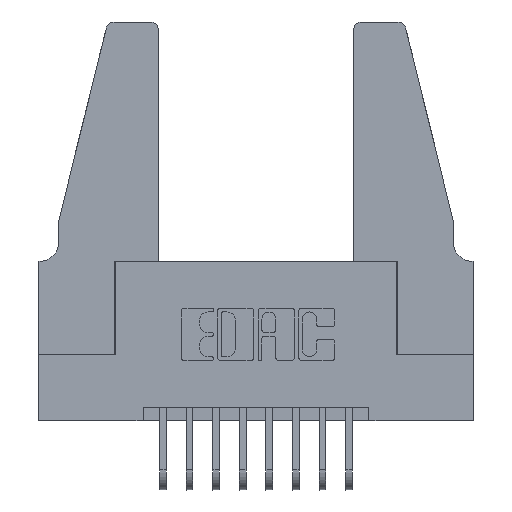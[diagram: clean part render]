
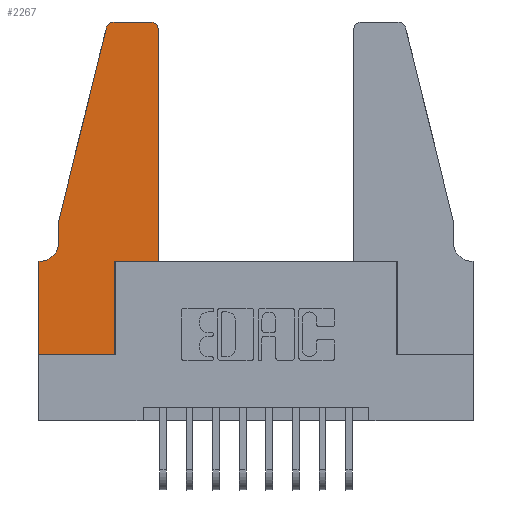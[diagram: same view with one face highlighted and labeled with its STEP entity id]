
A CAD part, top view. The second image highlights one B-rep face of the part: STEP entity #2267.
In plain terms, the highlighted planar face has unit normal (0, 0, 1).
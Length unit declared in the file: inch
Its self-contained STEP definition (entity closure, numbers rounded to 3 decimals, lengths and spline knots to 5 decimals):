
#106 = ORIENTED_EDGE ( 'NONE', *, *, #3151, .T. ) ;
#314 = VECTOR ( 'NONE', #9955, 39.37008 ) ;
#373 = CARTESIAN_POINT ( 'NONE',  ( 0.0755, 0.5, 0.37 ) ) ;
#495 = AXIS2_PLACEMENT_3D ( 'NONE', #718, #8712, #1900 ) ;
#718 = CARTESIAN_POINT ( 'NONE',  ( 0.284, 1.22, 0.37 ) ) ;
#794 = CARTESIAN_POINT ( 'NONE',  ( 0.4205, 1.25, 0.37 ) ) ;
#854 = EDGE_CURVE ( 'NONE', #6997, #4150, #3758, .T. ) ;
#911 = CARTESIAN_POINT ( 'NONE',  ( 0.0755, 0.42, 0.37 ) ) ;
#1144 = EDGE_CURVE ( 'NONE', #11547, #2242, #6611, .T. ) ;
#1324 = ORIENTED_EDGE ( 'NONE', *, *, #3667, .T. ) ;
#1721 = DIRECTION ( 'NONE',  ( 0., -1., 0. ) ) ;
#1776 = EDGE_CURVE ( 'NONE', #3511, #8217, #12428, .T. ) ;
#1794 = EDGE_CURVE ( 'NONE', #9923, #12854, #3394, .T. ) ;
#1900 = DIRECTION ( 'NONE',  ( 1., 0., 0. ) ) ;
#2242 = VERTEX_POINT ( 'NONE', #13448 ) ;
#2267 = ADVANCED_FACE ( 'NONE', ( #3714 ), #11878, .T. ) ;
#2472 = VECTOR ( 'NONE', #1721, 39.37008 ) ;
#3151 = EDGE_CURVE ( 'NONE', #4376, #7071, #13281, .T. ) ;
#3242 = AXIS2_PLACEMENT_3D ( 'NONE', #13270, #6522, #14371 ) ;
#3285 = CARTESIAN_POINT ( 'NONE',  ( 0.2865, 0., 0.37 ) ) ;
#3394 = LINE ( 'NONE', #8948, #9116 ) ;
#3441 = LINE ( 'NONE', #11958, #6100 ) ;
#3511 = VERTEX_POINT ( 'NONE', #8532 ) ;
#3667 = EDGE_CURVE ( 'NONE', #12217, #9923, #12231, .T. ) ;
#3714 = FACE_OUTER_BOUND ( 'NONE', #9520, .T. ) ;
#3758 = LINE ( 'NONE', #11644, #4121 ) ;
#3911 = DIRECTION ( 'NONE',  ( -1., 0., 0. ) ) ;
#3915 = ORIENTED_EDGE ( 'NONE', *, *, #9775, .T. ) ;
#4121 = VECTOR ( 'NONE', #10924, 39.37008 ) ;
#4150 = VERTEX_POINT ( 'NONE', #373 ) ;
#4205 = AXIS2_PLACEMENT_3D ( 'NONE', #7720, #7702, #7655 ) ;
#4224 = EDGE_CURVE ( 'NONE', #4759, #12217, #14110, .T. ) ;
#4376 = VERTEX_POINT ( 'NONE', #794 ) ;
#4382 = CARTESIAN_POINT ( 'NONE',  ( 0.2605, 1.25, 0.37 ) ) ;
#4759 = VERTEX_POINT ( 'NONE', #7159 ) ;
#4923 = ORIENTED_EDGE ( 'NONE', *, *, #854, .T. ) ;
#4986 = CIRCLE ( 'NONE', #3242, 0.03 ) ;
#5549 = ORIENTED_EDGE ( 'NONE', *, *, #1144, .T. ) ;
#5839 = VECTOR ( 'NONE', #13183, 39.37008 ) ;
#5898 = CARTESIAN_POINT ( 'NONE',  ( 0., 0., 0.37 ) ) ;
#5924 = VECTOR ( 'NONE', #11223, 39.37008 ) ;
#5945 = DIRECTION ( 'NONE',  ( 0., -1., 0. ) ) ;
#6098 = LINE ( 'NONE', #13817, #8793 ) ;
#6100 = VECTOR ( 'NONE', #6314, 39.37008 ) ;
#6314 = DIRECTION ( 'NONE',  ( 1., 0., 0. ) ) ;
#6492 = ORIENTED_EDGE ( 'NONE', *, *, #4224, .T. ) ;
#6522 = DIRECTION ( 'NONE',  ( 0., 0., 1. ) ) ;
#6611 = CIRCLE ( 'NONE', #4205, 0.07 ) ;
#6670 = CIRCLE ( 'NONE', #495, 0.03 ) ;
#6826 = EDGE_CURVE ( 'NONE', #12854, #3511, #3441, .T. ) ;
#6924 = VECTOR ( 'NONE', #3911, 39.37008 ) ;
#6997 = VERTEX_POINT ( 'NONE', #12692 ) ;
#7071 = VERTEX_POINT ( 'NONE', #7173 ) ;
#7159 = CARTESIAN_POINT ( 'NONE',  ( 0., 0.35, 0.37 ) ) ;
#7173 = CARTESIAN_POINT ( 'NONE',  ( 0.284, 1.25, 0.37 ) ) ;
#7655 = DIRECTION ( 'NONE',  ( -1., 0., 0. ) ) ;
#7702 = DIRECTION ( 'NONE',  ( 0., 0., -1. ) ) ;
#7720 = CARTESIAN_POINT ( 'NONE',  ( 0.0055, 0.42, 0.37 ) ) ;
#7837 = CARTESIAN_POINT ( 'NONE',  ( 0., 0., 0.37 ) ) ;
#7956 = DIRECTION ( 'NONE',  ( 0., 1., 0. ) ) ;
#8012 = CARTESIAN_POINT ( 'NONE',  ( 0.4505, 1.22, 0.37 ) ) ;
#8217 = VERTEX_POINT ( 'NONE', #8012 ) ;
#8532 = CARTESIAN_POINT ( 'NONE',  ( 0.4505, 0.35, 0.37 ) ) ;
#8537 = CARTESIAN_POINT ( 'NONE',  ( 0., 0., 0.37 ) ) ;
#8624 = LINE ( 'NONE', #10100, #5924 ) ;
#8635 = AXIS2_PLACEMENT_3D ( 'NONE', #11073, #11070, #11036 ) ;
#8712 = DIRECTION ( 'NONE',  ( 0., 0., 1. ) ) ;
#8793 = VECTOR ( 'NONE', #5945, 39.37008 ) ;
#8807 = ORIENTED_EDGE ( 'NONE', *, *, #6826, .T. ) ;
#8948 = CARTESIAN_POINT ( 'NONE',  ( 0.2865, 0.35, 0.37 ) ) ;
#9116 = VECTOR ( 'NONE', #7956, 39.37008 ) ;
#9520 = EDGE_LOOP ( 'NONE', ( #106, #3915, #4923, #14349, #5549, #10316, #6492, #1324, #13545, #8807, #11509, #13063 ) ) ;
#9533 = CARTESIAN_POINT ( 'NONE',  ( 0.2865, 0.35, 0.37 ) ) ;
#9772 = CARTESIAN_POINT ( 'NONE',  ( 0.4505, 0.35, 0.37 ) ) ;
#9775 = EDGE_CURVE ( 'NONE', #7071, #6997, #6670, .T. ) ;
#9923 = VERTEX_POINT ( 'NONE', #3285 ) ;
#9955 = DIRECTION ( 'NONE',  ( 0., 1., 0. ) ) ;
#10100 = CARTESIAN_POINT ( 'NONE',  ( 0.0755, 0.35, 0.37 ) ) ;
#10311 = EDGE_CURVE ( 'NONE', #2242, #4759, #8624, .T. ) ;
#10316 = ORIENTED_EDGE ( 'NONE', *, *, #10311, .T. ) ;
#10924 = DIRECTION ( 'NONE',  ( -0.239, -0.971, 0. ) ) ;
#11036 = DIRECTION ( 'NONE',  ( 1., 0., 0. ) ) ;
#11070 = DIRECTION ( 'NONE',  ( 0., 0., 1. ) ) ;
#11073 = CARTESIAN_POINT ( 'NONE',  ( 0., 0.35, 0.37 ) ) ;
#11216 = EDGE_CURVE ( 'NONE', #4150, #11547, #6098, .T. ) ;
#11223 = DIRECTION ( 'NONE',  ( -1., 0., 0. ) ) ;
#11509 = ORIENTED_EDGE ( 'NONE', *, *, #1776, .T. ) ;
#11547 = VERTEX_POINT ( 'NONE', #911 ) ;
#11644 = CARTESIAN_POINT ( 'NONE',  ( 0.0755, 0.5, 0.37 ) ) ;
#11878 = PLANE ( 'NONE',  #8635 ) ;
#11958 = CARTESIAN_POINT ( 'NONE',  ( 0.4505, 0.35, 0.37 ) ) ;
#12217 = VERTEX_POINT ( 'NONE', #7837 ) ;
#12231 = LINE ( 'NONE', #5898, #5839 ) ;
#12428 = LINE ( 'NONE', #9772, #314 ) ;
#12620 = EDGE_CURVE ( 'NONE', #8217, #4376, #4986, .T. ) ;
#12692 = CARTESIAN_POINT ( 'NONE',  ( 0.25487, 1.22718, 0.37 ) ) ;
#12854 = VERTEX_POINT ( 'NONE', #9533 ) ;
#13063 = ORIENTED_EDGE ( 'NONE', *, *, #12620, .T. ) ;
#13183 = DIRECTION ( 'NONE',  ( 1., 0., 0. ) ) ;
#13270 = CARTESIAN_POINT ( 'NONE',  ( 0.4205, 1.22, 0.37 ) ) ;
#13281 = LINE ( 'NONE', #4382, #6924 ) ;
#13448 = CARTESIAN_POINT ( 'NONE',  ( 0.0055, 0.35, 0.37 ) ) ;
#13545 = ORIENTED_EDGE ( 'NONE', *, *, #1794, .T. ) ;
#13817 = CARTESIAN_POINT ( 'NONE',  ( 0.0755, 0.5, 0.37 ) ) ;
#14110 = LINE ( 'NONE', #8537, #2472 ) ;
#14349 = ORIENTED_EDGE ( 'NONE', *, *, #11216, .T. ) ;
#14371 = DIRECTION ( 'NONE',  ( 1., 0., 0. ) ) ;
